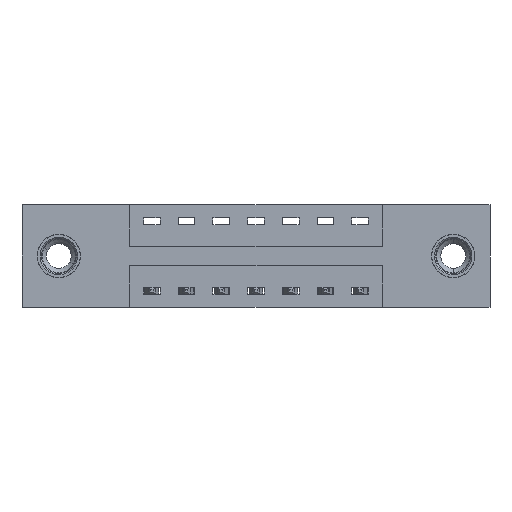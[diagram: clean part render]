
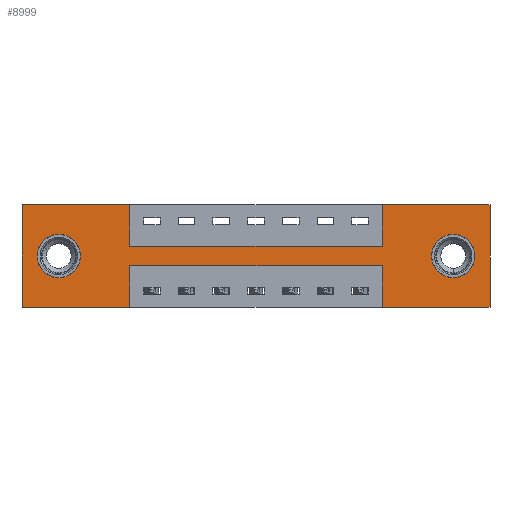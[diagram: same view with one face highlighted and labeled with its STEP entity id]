
A CAD part, front view. The second image highlights one B-rep face of the part: STEP entity #8999.
In plain terms, the highlighted planar face has unit normal (0, -1, 0).
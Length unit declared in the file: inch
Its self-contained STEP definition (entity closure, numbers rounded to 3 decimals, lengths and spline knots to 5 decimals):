
#143 = DIRECTION ( 'NONE',  ( 0., 0., -1. ) ) ;
#396 = CARTESIAN_POINT ( 'NONE',  ( 1.5525, 0., -0.107 ) ) ;
#484 = VECTOR ( 'NONE', #8609, 39.37008 ) ;
#486 = VECTOR ( 'NONE', #6528, 39.37008 ) ;
#520 = CARTESIAN_POINT ( 'NONE',  ( 0., 0., 0. ) ) ;
#548 = VERTEX_POINT ( 'NONE', #3499 ) ;
#616 = CARTESIAN_POINT ( 'NONE',  ( 1.2975, 0., -0.37 ) ) ;
#682 = ORIENTED_EDGE ( 'NONE', *, *, #2039, .F. ) ;
#702 = ORIENTED_EDGE ( 'NONE', *, *, #2302, .F. ) ;
#762 = LINE ( 'NONE', #5740, #486 ) ;
#906 = VECTOR ( 'NONE', #2872, 39.37008 ) ;
#990 = EDGE_CURVE ( 'NONE', #5620, #1503, #4809, .T. ) ;
#1124 = EDGE_CURVE ( 'NONE', #1503, #5620, #1706, .T. ) ;
#1171 = CARTESIAN_POINT ( 'NONE',  ( 1.2975, 0., 0. ) ) ;
#1261 = CARTESIAN_POINT ( 'NONE',  ( 1.2975, 0., -0.37 ) ) ;
#1316 = CARTESIAN_POINT ( 'NONE',  ( 1.2975, 0., -0.22 ) ) ;
#1341 = ORIENTED_EDGE ( 'NONE', *, *, #990, .T. ) ;
#1350 = LINE ( 'NONE', #520, #2994 ) ;
#1382 = VERTEX_POINT ( 'NONE', #6932 ) ;
#1420 = ORIENTED_EDGE ( 'NONE', *, *, #7321, .F. ) ;
#1462 = VERTEX_POINT ( 'NONE', #1261 ) ;
#1503 = VERTEX_POINT ( 'NONE', #5994 ) ;
#1572 = CARTESIAN_POINT ( 'NONE',  ( 1.685, 0., 0. ) ) ;
#1660 = ORIENTED_EDGE ( 'NONE', *, *, #4663, .F. ) ;
#1706 = CIRCLE ( 'NONE', #8084, 0.078 ) ;
#1766 = DIRECTION ( 'NONE',  ( 0., 0., -1. ) ) ;
#1781 = LINE ( 'NONE', #2669, #3969 ) ;
#1856 = DIRECTION ( 'NONE',  ( 0., 0., -1. ) ) ;
#2039 = EDGE_CURVE ( 'NONE', #1462, #6247, #5768, .T. ) ;
#2045 = CARTESIAN_POINT ( 'NONE',  ( 1.685, 0., 0. ) ) ;
#2079 = ORIENTED_EDGE ( 'NONE', *, *, #8290, .F. ) ;
#2132 = CARTESIAN_POINT ( 'NONE',  ( 0.1325, 0., -0.185 ) ) ;
#2229 = FACE_BOUND ( 'NONE', #5005, .T. ) ;
#2302 = EDGE_CURVE ( 'NONE', #8593, #9725, #7467, .T. ) ;
#2626 = LINE ( 'NONE', #7849, #484 ) ;
#2655 = LINE ( 'NONE', #9128, #8991 ) ;
#2669 = CARTESIAN_POINT ( 'NONE',  ( 0., 0., -0.37 ) ) ;
#2698 = DIRECTION ( 'NONE',  ( -1., 0., 0. ) ) ;
#2872 = DIRECTION ( 'NONE',  ( 0., 0., -1. ) ) ;
#2873 = CARTESIAN_POINT ( 'NONE',  ( 0.3875, 0., -0.15 ) ) ;
#2957 = DIRECTION ( 'NONE',  ( 0., 0., 1. ) ) ;
#2975 = ORIENTED_EDGE ( 'NONE', *, *, #9765, .F. ) ;
#2994 = VECTOR ( 'NONE', #6179, 39.37008 ) ;
#3156 = EDGE_CURVE ( 'NONE', #8344, #4284, #1781, .T. ) ;
#3249 = CARTESIAN_POINT ( 'NONE',  ( 0.1325, 0., -0.185 ) ) ;
#3255 = VERTEX_POINT ( 'NONE', #1171 ) ;
#3386 = CARTESIAN_POINT ( 'NONE',  ( 0.3875, 0., 0. ) ) ;
#3409 = EDGE_CURVE ( 'NONE', #4804, #6709, #4082, .T. ) ;
#3478 = CARTESIAN_POINT ( 'NONE',  ( 1.2975, 0., -0.15 ) ) ;
#3499 = CARTESIAN_POINT ( 'NONE',  ( 1.685, 0., -0.37 ) ) ;
#3607 = VECTOR ( 'NONE', #3987, 39.37008 ) ;
#3623 = VERTEX_POINT ( 'NONE', #1572 ) ;
#3631 = DIRECTION ( 'NONE',  ( 0., 0., 1. ) ) ;
#3760 = CIRCLE ( 'NONE', #7986, 0.078 ) ;
#3919 = CARTESIAN_POINT ( 'NONE',  ( 0.3875, 0., -0.22 ) ) ;
#3956 = EDGE_CURVE ( 'NONE', #3623, #548, #5218, .T. ) ;
#3969 = VECTOR ( 'NONE', #5910, 39.37008 ) ;
#3987 = DIRECTION ( 'NONE',  ( 0., 0., 1. ) ) ;
#4057 = CARTESIAN_POINT ( 'NONE',  ( 1.5525, 0., -0.185 ) ) ;
#4066 = DIRECTION ( 'NONE',  ( 0., 0., 1. ) ) ;
#4082 = CIRCLE ( 'NONE', #8599, 0.078 ) ;
#4284 = VERTEX_POINT ( 'NONE', #8176 ) ;
#4475 = EDGE_CURVE ( 'NONE', #9725, #3255, #2655, .T. ) ;
#4482 = ORIENTED_EDGE ( 'NONE', *, *, #4475, .F. ) ;
#4663 = EDGE_CURVE ( 'NONE', #6247, #5092, #9103, .T. ) ;
#4804 = VERTEX_POINT ( 'NONE', #7356 ) ;
#4809 = CIRCLE ( 'NONE', #7050, 0.078 ) ;
#4844 = CARTESIAN_POINT ( 'NONE',  ( 0.3875, 0., -0.15 ) ) ;
#4873 = DIRECTION ( 'NONE',  ( 0., 0., -1. ) ) ;
#4876 = DIRECTION ( 'NONE',  ( 1., 0., 0. ) ) ;
#4969 = VECTOR ( 'NONE', #8631, 39.37008 ) ;
#5005 = EDGE_LOOP ( 'NONE', ( #1341, #9910 ) ) ;
#5019 = PLANE ( 'NONE',  #7193 ) ;
#5020 = DIRECTION ( 'NONE',  ( 0., 1., 0. ) ) ;
#5092 = VERTEX_POINT ( 'NONE', #10024 ) ;
#5163 = LINE ( 'NONE', #8984, #9052 ) ;
#5218 = LINE ( 'NONE', #2045, #906 ) ;
#5224 = ORIENTED_EDGE ( 'NONE', *, *, #7623, .F. ) ;
#5620 = VERTEX_POINT ( 'NONE', #396 ) ;
#5657 = ORIENTED_EDGE ( 'NONE', *, *, #8493, .F. ) ;
#5740 = CARTESIAN_POINT ( 'NONE',  ( 0., 0., 0. ) ) ;
#5768 = LINE ( 'NONE', #616, #3607 ) ;
#5826 = CARTESIAN_POINT ( 'NONE',  ( 0., 0., -0.37 ) ) ;
#5910 = DIRECTION ( 'NONE',  ( -1., 0., 0. ) ) ;
#5994 = CARTESIAN_POINT ( 'NONE',  ( 1.5525, 0., -0.263 ) ) ;
#6179 = DIRECTION ( 'NONE',  ( 1., 0., 0. ) ) ;
#6247 = VERTEX_POINT ( 'NONE', #1316 ) ;
#6296 = FACE_OUTER_BOUND ( 'NONE', #8457, .T. ) ;
#6528 = DIRECTION ( 'NONE',  ( 0., 0., 1. ) ) ;
#6594 = CARTESIAN_POINT ( 'NONE',  ( 0.3875, 0., -0.37 ) ) ;
#6609 = DIRECTION ( 'NONE',  ( 0., -1., 0. ) ) ;
#6709 = VERTEX_POINT ( 'NONE', #6766 ) ;
#6766 = CARTESIAN_POINT ( 'NONE',  ( 0.1325, 0., -0.263 ) ) ;
#6885 = EDGE_CURVE ( 'NONE', #3255, #3623, #1350, .T. ) ;
#6932 = CARTESIAN_POINT ( 'NONE',  ( 0., 0., 0. ) ) ;
#7016 = VECTOR ( 'NONE', #2698, 39.37008 ) ;
#7050 = AXIS2_PLACEMENT_3D ( 'NONE', #4057, #9546, #4873 ) ;
#7055 = VECTOR ( 'NONE', #9070, 39.37008 ) ;
#7193 = AXIS2_PLACEMENT_3D ( 'NONE', #5826, #6609, #1766 ) ;
#7321 = EDGE_CURVE ( 'NONE', #548, #1462, #9540, .T. ) ;
#7356 = CARTESIAN_POINT ( 'NONE',  ( 0.1325, 0., -0.107 ) ) ;
#7467 = LINE ( 'NONE', #4844, #9263 ) ;
#7507 = CARTESIAN_POINT ( 'NONE',  ( 0., 0., -0.37 ) ) ;
#7623 = EDGE_CURVE ( 'NONE', #5092, #8344, #2626, .T. ) ;
#7751 = DIRECTION ( 'NONE',  ( 0., 1., 0. ) ) ;
#7805 = EDGE_LOOP ( 'NONE', ( #8664, #8164 ) ) ;
#7849 = CARTESIAN_POINT ( 'NONE',  ( 0.3875, 0., -0.37 ) ) ;
#7986 = AXIS2_PLACEMENT_3D ( 'NONE', #3249, #8773, #4066 ) ;
#8084 = AXIS2_PLACEMENT_3D ( 'NONE', #9678, #5020, #143 ) ;
#8164 = ORIENTED_EDGE ( 'NONE', *, *, #10135, .T. ) ;
#8176 = CARTESIAN_POINT ( 'NONE',  ( 0., 0., -0.37 ) ) ;
#8290 = EDGE_CURVE ( 'NONE', #4284, #1382, #762, .T. ) ;
#8309 = CARTESIAN_POINT ( 'NONE',  ( 0., 0., 0. ) ) ;
#8344 = VERTEX_POINT ( 'NONE', #6594 ) ;
#8457 = EDGE_LOOP ( 'NONE', ( #5224, #1660, #682, #1420, #9517, #9991, #4482, #702, #2975, #5657, #2079, #10142 ) ) ;
#8493 = EDGE_CURVE ( 'NONE', #1382, #8986, #9077, .T. ) ;
#8593 = VERTEX_POINT ( 'NONE', #2873 ) ;
#8599 = AXIS2_PLACEMENT_3D ( 'NONE', #2132, #7751, #2957 ) ;
#8609 = DIRECTION ( 'NONE',  ( 0., 0., -1. ) ) ;
#8631 = DIRECTION ( 'NONE',  ( -1., 0., 0. ) ) ;
#8664 = ORIENTED_EDGE ( 'NONE', *, *, #3409, .T. ) ;
#8773 = DIRECTION ( 'NONE',  ( 0., 1., 0. ) ) ;
#8984 = CARTESIAN_POINT ( 'NONE',  ( 0.3875, 0., 0. ) ) ;
#8986 = VERTEX_POINT ( 'NONE', #3386 ) ;
#8991 = VECTOR ( 'NONE', #3631, 39.37008 ) ;
#8999 = ADVANCED_FACE ( 'NONE', ( #2229, #10152, #6296 ), #5019, .T. ) ;
#9052 = VECTOR ( 'NONE', #1856, 39.37008 ) ;
#9070 = DIRECTION ( 'NONE',  ( 1., 0., 0. ) ) ;
#9077 = LINE ( 'NONE', #8309, #7055 ) ;
#9103 = LINE ( 'NONE', #3919, #4969 ) ;
#9128 = CARTESIAN_POINT ( 'NONE',  ( 1.2975, 0., 0. ) ) ;
#9263 = VECTOR ( 'NONE', #4876, 39.37008 ) ;
#9517 = ORIENTED_EDGE ( 'NONE', *, *, #3956, .F. ) ;
#9540 = LINE ( 'NONE', #7507, #7016 ) ;
#9546 = DIRECTION ( 'NONE',  ( 0., 1., 0. ) ) ;
#9678 = CARTESIAN_POINT ( 'NONE',  ( 1.5525, 0., -0.185 ) ) ;
#9725 = VERTEX_POINT ( 'NONE', #3478 ) ;
#9765 = EDGE_CURVE ( 'NONE', #8986, #8593, #5163, .T. ) ;
#9910 = ORIENTED_EDGE ( 'NONE', *, *, #1124, .T. ) ;
#9991 = ORIENTED_EDGE ( 'NONE', *, *, #6885, .F. ) ;
#10024 = CARTESIAN_POINT ( 'NONE',  ( 0.3875, 0., -0.22 ) ) ;
#10135 = EDGE_CURVE ( 'NONE', #6709, #4804, #3760, .T. ) ;
#10142 = ORIENTED_EDGE ( 'NONE', *, *, #3156, .F. ) ;
#10152 = FACE_BOUND ( 'NONE', #7805, .T. ) ;
